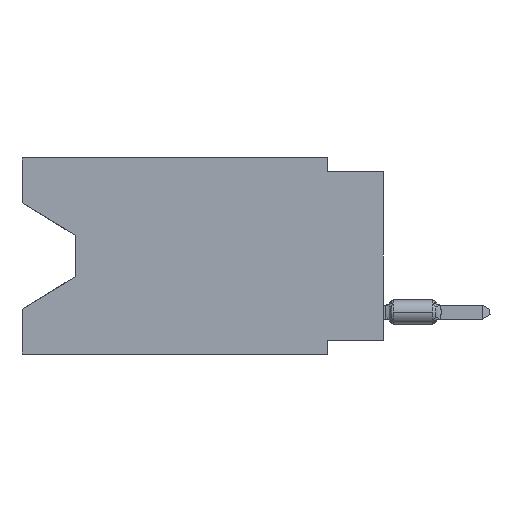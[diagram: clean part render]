
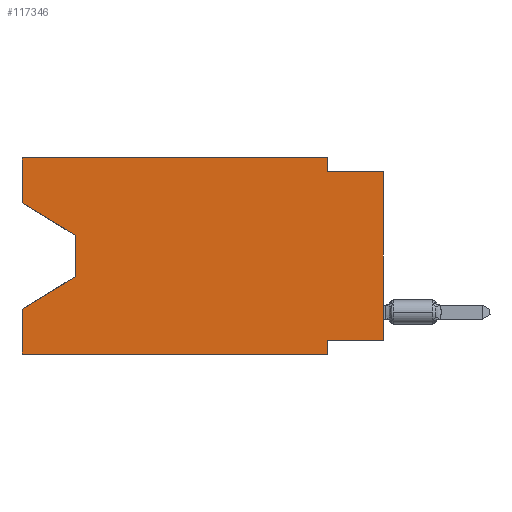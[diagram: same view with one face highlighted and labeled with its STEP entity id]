
A CAD part, left-side view. The second image highlights one B-rep face of the part: STEP entity #117346.
In plain terms, the highlighted planar face has unit normal (-1, 0, 0).
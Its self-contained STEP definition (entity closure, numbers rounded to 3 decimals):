
#153 = VERTEX_POINT ( 'NONE', #36325 ) ;
#1992 = LINE ( 'NONE', #13429, #2816 ) ;
#2362 = VERTEX_POINT ( 'NONE', #86912 ) ;
#2816 = VECTOR ( 'NONE', #50260, 1000. ) ;
#2887 = EDGE_CURVE ( 'NONE', #22322, #103909, #51762, .T. ) ;
#5093 = EDGE_CURVE ( 'NONE', #153, #50539, #83382, .T. ) ;
#5856 = VERTEX_POINT ( 'NONE', #76384 ) ;
#6157 = CARTESIAN_POINT ( 'NONE',  ( 0., 16.383, -2.038 ) ) ;
#6264 = LINE ( 'NONE', #26159, #8531 ) ;
#7573 = ORIENTED_EDGE ( 'NONE', *, *, #36272, .F. ) ;
#8531 = VECTOR ( 'NONE', #43078, 1000. ) ;
#10301 = CARTESIAN_POINT ( 'NONE',  ( 0., 13.97, -3.505 ) ) ;
#10510 = ORIENTED_EDGE ( 'NONE', *, *, #75916, .F. ) ;
#12305 = VECTOR ( 'NONE', #38146, 1000. ) ;
#13429 = CARTESIAN_POINT ( 'NONE',  ( 0., 13.97, -5.385 ) ) ;
#13726 = DIRECTION ( 'NONE',  ( 0., -0.855, -0.519 ) ) ;
#14939 = CARTESIAN_POINT ( 'NONE',  ( 0., 13.97, -3.505 ) ) ;
#15042 = LINE ( 'NONE', #88077, #20972 ) ;
#15531 = DIRECTION ( 'NONE',  ( 0., 0., -1. ) ) ;
#17615 = DIRECTION ( 'NONE',  ( 0., 0., -1. ) ) ;
#18567 = ORIENTED_EDGE ( 'NONE', *, *, #5093, .F. ) ;
#18629 = DIRECTION ( 'NONE',  ( 0., 0., -1. ) ) ;
#19166 = CARTESIAN_POINT ( 'NONE',  ( 0., 2.54, 0. ) ) ;
#20972 = VECTOR ( 'NONE', #22333, 1000. ) ;
#21115 = VERTEX_POINT ( 'NONE', #104463 ) ;
#21445 = VECTOR ( 'NONE', #13726, 1000. ) ;
#22322 = VERTEX_POINT ( 'NONE', #10301 ) ;
#22333 = DIRECTION ( 'NONE',  ( 0., 0., 1. ) ) ;
#22792 = LINE ( 'NONE', #31859, #21445 ) ;
#23972 = VECTOR ( 'NONE', #59849, 1000. ) ;
#25337 = ORIENTED_EDGE ( 'NONE', *, *, #71310, .T. ) ;
#26159 = CARTESIAN_POINT ( 'NONE',  ( 0., 0., -8.255 ) ) ;
#27166 = CARTESIAN_POINT ( 'NONE',  ( 0., 2.54, -8.255 ) ) ;
#29542 = CARTESIAN_POINT ( 'NONE',  ( 0., 13.97, -5.385 ) ) ;
#31502 = LINE ( 'NONE', #49638, #23972 ) ;
#31859 = CARTESIAN_POINT ( 'NONE',  ( 0., 16.383, -2.038 ) ) ;
#34880 = VECTOR ( 'NONE', #17615, 1000. ) ;
#35796 = VECTOR ( 'NONE', #100302, 1000. ) ;
#36272 = EDGE_CURVE ( 'NONE', #81981, #61993, #56039, .T. ) ;
#36325 = CARTESIAN_POINT ( 'NONE',  ( 0., 2.54, -0.635 ) ) ;
#38146 = DIRECTION ( 'NONE',  ( 0., 0., 1. ) ) ;
#38242 = CARTESIAN_POINT ( 'NONE',  ( 0., 2.54, -8.89 ) ) ;
#41281 = ORIENTED_EDGE ( 'NONE', *, *, #87157, .F. ) ;
#43078 = DIRECTION ( 'NONE',  ( 0., 1., 0. ) ) ;
#44792 = LINE ( 'NONE', #64073, #83040 ) ;
#44821 = EDGE_CURVE ( 'NONE', #2362, #81981, #6264, .T. ) ;
#44892 = EDGE_CURVE ( 'NONE', #21115, #61993, #31502, .T. ) ;
#47170 = CARTESIAN_POINT ( 'NONE',  ( 0., 2.54, 0. ) ) ;
#48711 = PLANE ( 'NONE',  #83401 ) ;
#49638 = CARTESIAN_POINT ( 'NONE',  ( 0., 16.383, -8.89 ) ) ;
#50260 = DIRECTION ( 'NONE',  ( 0., 0.855, -0.519 ) ) ;
#50539 = VERTEX_POINT ( 'NONE', #117041 ) ;
#51762 = LINE ( 'NONE', #14939, #118586 ) ;
#56039 = LINE ( 'NONE', #111541, #99024 ) ;
#57125 = ORIENTED_EDGE ( 'NONE', *, *, #44821, .F. ) ;
#58350 = CARTESIAN_POINT ( 'NONE',  ( 0., 16.383, 0. ) ) ;
#59849 = DIRECTION ( 'NONE',  ( 0., -1., 0. ) ) ;
#60545 = VECTOR ( 'NONE', #116900, 1000. ) ;
#61396 = CARTESIAN_POINT ( 'NONE',  ( 0., 16.383, 0. ) ) ;
#61993 = VERTEX_POINT ( 'NONE', #38242 ) ;
#62174 = EDGE_LOOP ( 'NONE', ( #25337, #86257, #111717, #90368, #99123, #7573, #57125, #106605, #18567, #88197, #41281, #10510 ) ) ;
#63488 = CARTESIAN_POINT ( 'NONE',  ( 0., 0., -0.635 ) ) ;
#63521 = EDGE_CURVE ( 'NONE', #2362, #50539, #44792, .T. ) ;
#63522 = EDGE_CURVE ( 'NONE', #83743, #153, #100884, .T. ) ;
#64073 = CARTESIAN_POINT ( 'NONE',  ( 0., 0., 0. ) ) ;
#65004 = FACE_OUTER_BOUND ( 'NONE', #62174, .T. ) ;
#69259 = LINE ( 'NONE', #61396, #60545 ) ;
#71310 = EDGE_CURVE ( 'NONE', #112185, #22322, #22792, .T. ) ;
#73726 = DIRECTION ( 'NONE',  ( 0., 0., 1. ) ) ;
#74657 = DIRECTION ( 'NONE',  ( 1., 0., 0. ) ) ;
#74887 = VERTEX_POINT ( 'NONE', #88733 ) ;
#75542 = LINE ( 'NONE', #112333, #12305 ) ;
#75916 = EDGE_CURVE ( 'NONE', #112185, #74887, #75542, .T. ) ;
#76384 = CARTESIAN_POINT ( 'NONE',  ( 0., 16.383, -6.852 ) ) ;
#81981 = VERTEX_POINT ( 'NONE', #27166 ) ;
#83040 = VECTOR ( 'NONE', #73726, 1000. ) ;
#83382 = LINE ( 'NONE', #63488, #35796 ) ;
#83401 = AXIS2_PLACEMENT_3D ( 'NONE', #58350, #74657, #93958 ) ;
#83743 = VERTEX_POINT ( 'NONE', #19166 ) ;
#86257 = ORIENTED_EDGE ( 'NONE', *, *, #2887, .T. ) ;
#86912 = CARTESIAN_POINT ( 'NONE',  ( 0., 0., -8.255 ) ) ;
#87157 = EDGE_CURVE ( 'NONE', #74887, #83743, #69259, .T. ) ;
#88077 = CARTESIAN_POINT ( 'NONE',  ( 0., 16.383, 0. ) ) ;
#88197 = ORIENTED_EDGE ( 'NONE', *, *, #63522, .F. ) ;
#88733 = CARTESIAN_POINT ( 'NONE',  ( 0., 16.383, 0. ) ) ;
#90368 = ORIENTED_EDGE ( 'NONE', *, *, #92604, .F. ) ;
#92604 = EDGE_CURVE ( 'NONE', #21115, #5856, #15042, .T. ) ;
#93958 = DIRECTION ( 'NONE',  ( 0., 0., -1. ) ) ;
#97171 = EDGE_CURVE ( 'NONE', #103909, #5856, #1992, .T. ) ;
#99024 = VECTOR ( 'NONE', #18629, 1000. ) ;
#99123 = ORIENTED_EDGE ( 'NONE', *, *, #44892, .T. ) ;
#100302 = DIRECTION ( 'NONE',  ( 0., -1., 0. ) ) ;
#100884 = LINE ( 'NONE', #47170, #34880 ) ;
#103909 = VERTEX_POINT ( 'NONE', #29542 ) ;
#104463 = CARTESIAN_POINT ( 'NONE',  ( 0., 16.383, -8.89 ) ) ;
#106605 = ORIENTED_EDGE ( 'NONE', *, *, #63521, .T. ) ;
#111541 = CARTESIAN_POINT ( 'NONE',  ( 0., 2.54, -8.89 ) ) ;
#111717 = ORIENTED_EDGE ( 'NONE', *, *, #97171, .T. ) ;
#112185 = VERTEX_POINT ( 'NONE', #6157 ) ;
#112333 = CARTESIAN_POINT ( 'NONE',  ( 0., 16.383, 0. ) ) ;
#116900 = DIRECTION ( 'NONE',  ( 0., -1., 0. ) ) ;
#117041 = CARTESIAN_POINT ( 'NONE',  ( 0., 0., -0.635 ) ) ;
#117346 = ADVANCED_FACE ( 'NONE', ( #65004 ), #48711, .F. ) ;
#118586 = VECTOR ( 'NONE', #15531, 1000. ) ;
